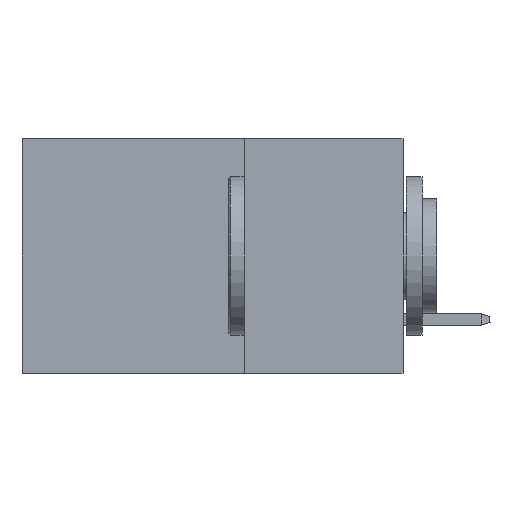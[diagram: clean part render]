
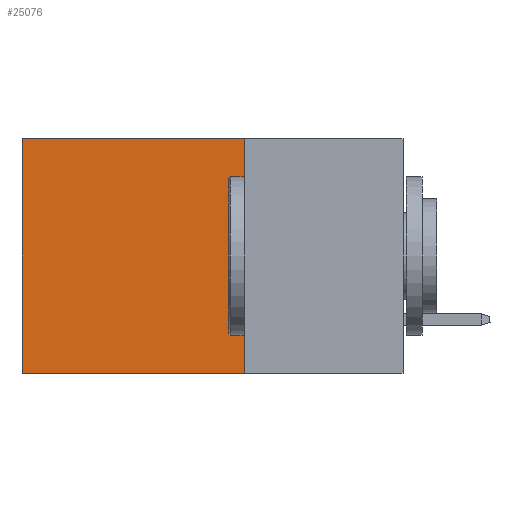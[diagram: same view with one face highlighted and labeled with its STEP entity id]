
A CAD part, left-side view. The second image highlights one B-rep face of the part: STEP entity #25076.
In plain terms, the highlighted planar face has unit normal (-1, 0, 0).
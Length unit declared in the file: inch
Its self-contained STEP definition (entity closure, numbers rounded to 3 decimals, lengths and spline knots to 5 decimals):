
#217 = AXIS2_PLACEMENT_3D ( 'NONE', #9266, #17531, #25817 ) ;
#979 = PLANE ( 'NONE',  #217 ) ;
#3051 = VERTEX_POINT ( 'NONE', #6078 ) ;
#3689 = EDGE_CURVE ( 'NONE', #17538, #8173, #13877, .T. ) ;
#4091 = EDGE_LOOP ( 'NONE', ( #18160, #14494, #9277, #21617 ) ) ;
#4611 = CARTESIAN_POINT ( 'NONE',  ( 0.2875, 0.25, 0. ) ) ;
#6078 = CARTESIAN_POINT ( 'NONE',  ( 0.2875, 0.25, 0. ) ) ;
#6545 = CARTESIAN_POINT ( 'NONE',  ( 0.2875, 0.6, 0. ) ) ;
#7999 = CARTESIAN_POINT ( 'NONE',  ( 0.2875, 0.25, 0. ) ) ;
#8173 = VERTEX_POINT ( 'NONE', #22349 ) ;
#8270 = LINE ( 'NONE', #4611, #13246 ) ;
#9266 = CARTESIAN_POINT ( 'NONE',  ( 0.2875, 0.25, 0. ) ) ;
#9277 = ORIENTED_EDGE ( 'NONE', *, *, #26182, .F. ) ;
#10085 = EDGE_CURVE ( 'NONE', #3051, #17538, #24422, .T. ) ;
#10214 = DIRECTION ( 'NONE',  ( 0., 0., -1. ) ) ;
#11292 = FACE_OUTER_BOUND ( 'NONE', #4091, .T. ) ;
#11820 = EDGE_CURVE ( 'NONE', #21270, #8173, #22087, .T. ) ;
#12868 = DIRECTION ( 'NONE',  ( 0., 0., -1. ) ) ;
#13246 = VECTOR ( 'NONE', #12868, 39.37008 ) ;
#13740 = CARTESIAN_POINT ( 'NONE',  ( 0.2875, 0.6, 0. ) ) ;
#13877 = LINE ( 'NONE', #13740, #20111 ) ;
#14494 = ORIENTED_EDGE ( 'NONE', *, *, #11820, .F. ) ;
#17531 = DIRECTION ( 'NONE',  ( 1., 0., 0. ) ) ;
#17538 = VERTEX_POINT ( 'NONE', #6545 ) ;
#18160 = ORIENTED_EDGE ( 'NONE', *, *, #3689, .T. ) ;
#18409 = DIRECTION ( 'NONE',  ( 0., 1., 0. ) ) ;
#18527 = CARTESIAN_POINT ( 'NONE',  ( 0.2875, 0.25, -0.37 ) ) ;
#18635 = VECTOR ( 'NONE', #26180, 39.37008 ) ;
#20111 = VECTOR ( 'NONE', #10214, 39.37008 ) ;
#21270 = VERTEX_POINT ( 'NONE', #25391 ) ;
#21617 = ORIENTED_EDGE ( 'NONE', *, *, #10085, .T. ) ;
#22087 = LINE ( 'NONE', #18527, #22429 ) ;
#22349 = CARTESIAN_POINT ( 'NONE',  ( 0.2875, 0.6, -0.37 ) ) ;
#22429 = VECTOR ( 'NONE', #18409, 39.37008 ) ;
#24422 = LINE ( 'NONE', #7999, #18635 ) ;
#25076 = ADVANCED_FACE ( 'NONE', ( #11292 ), #979, .F. ) ;
#25391 = CARTESIAN_POINT ( 'NONE',  ( 0.2875, 0.25, -0.37 ) ) ;
#25817 = DIRECTION ( 'NONE',  ( 0., 0., -1. ) ) ;
#26180 = DIRECTION ( 'NONE',  ( 0., 1., 0. ) ) ;
#26182 = EDGE_CURVE ( 'NONE', #3051, #21270, #8270, .T. ) ;
